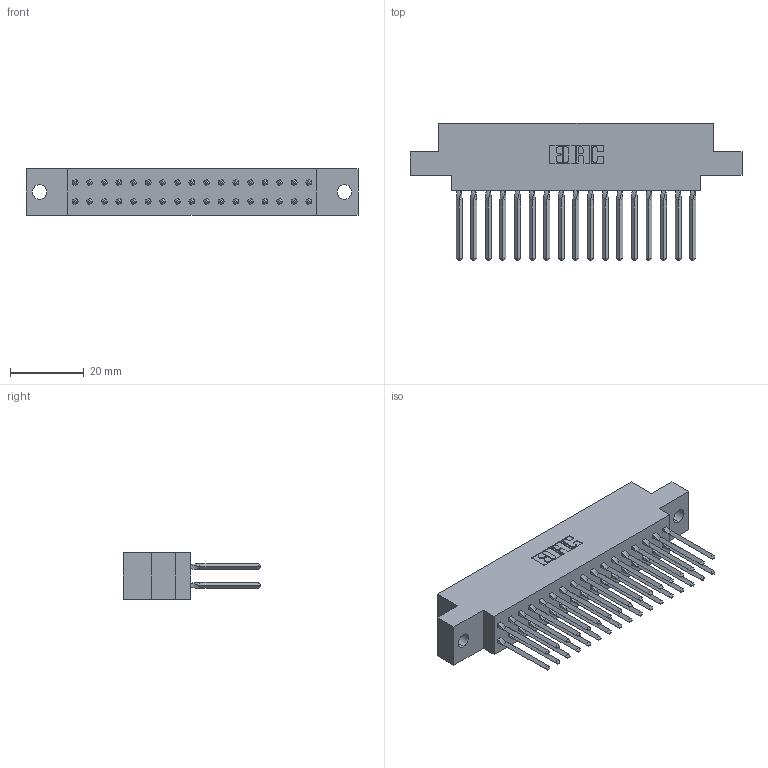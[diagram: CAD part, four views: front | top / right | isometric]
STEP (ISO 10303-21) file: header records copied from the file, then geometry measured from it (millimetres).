
FILE_DESCRIPTION (( 'STEP AP203' ), '1' );
FILE_NAME ('317-034-540-804.STEP', '2020-02-27T21:56:11', ( '' ), ( '' ), 'SwSTEP 2.0', 'SolidWorks 2016', '' );
FILE_SCHEMA (( 'CONFIG_CONTROL_DESIGN' ));
Length unit declared in the file: inch
Products named in the file (3): 317-034-540-804; 317 Part_.156 Dia - TH; 317-290-001_540
Assembly tree (35 placements, depth 2):
  317-034-540-804
    317 Part_.156 Dia - TH
    317-290-001_540  x34
Bounding box: 90.07 x 37.34 x 12.7 mm (x, y, z)
Volume: 14183.1 mm3; surface area: 20026.5 mm2
Topology: 35 solids, 35 shells, 3128 faces, 8673 edges, 5588 vertices
Faces by surface type: plane 2540, cylinder 452, bspline 136
Entity records: 28064 total; most frequent: CARTESIAN_POINT 5307, ORIENTED_EDGE 4806, DIRECTION 4013, EDGE_CURVE 2403, LINE 2147, VECTOR 2147, VERTEX_POINT 1595, AXIS2_PLACEMENT_3D 933
